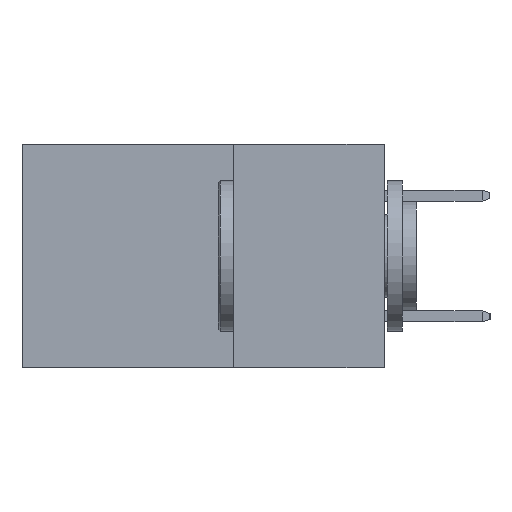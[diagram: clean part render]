
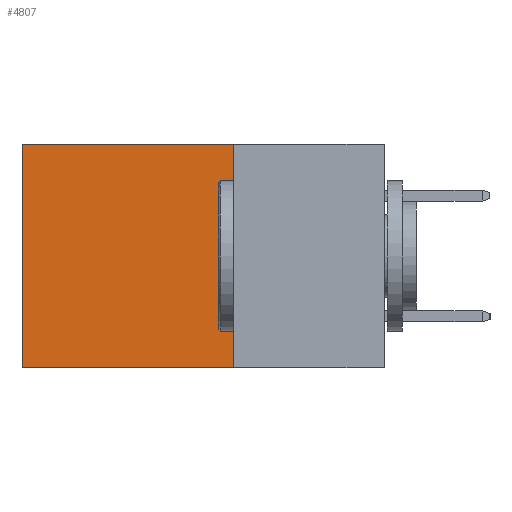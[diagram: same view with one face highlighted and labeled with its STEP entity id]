
A CAD part, left-side view. The second image highlights one B-rep face of the part: STEP entity #4807.
In plain terms, the highlighted planar face has unit normal (-1, 0, 0).
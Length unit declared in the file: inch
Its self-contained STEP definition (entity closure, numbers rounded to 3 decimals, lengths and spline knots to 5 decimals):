
#549 = EDGE_LOOP ( 'NONE', ( #6745, #1551, #2365, #1189 ) ) ;
#686 = DIRECTION ( 'NONE',  ( 0., 1., 0. ) ) ;
#787 = CARTESIAN_POINT ( 'NONE',  ( 0.2615, 0.25, 0. ) ) ;
#834 = FACE_OUTER_BOUND ( 'NONE', #549, .T. ) ;
#1189 = ORIENTED_EDGE ( 'NONE', *, *, #6927, .T. ) ;
#1272 = LINE ( 'NONE', #2302, #10806 ) ;
#1416 = CARTESIAN_POINT ( 'NONE',  ( 0.2615, 0.6, 0. ) ) ;
#1425 = AXIS2_PLACEMENT_3D ( 'NONE', #8714, #7562, #7513 ) ;
#1551 = ORIENTED_EDGE ( 'NONE', *, *, #2370, .F. ) ;
#2302 = CARTESIAN_POINT ( 'NONE',  ( 0.2615, 0.25, -0.37 ) ) ;
#2365 = ORIENTED_EDGE ( 'NONE', *, *, #4646, .F. ) ;
#2370 = EDGE_CURVE ( 'NONE', #10012, #10763, #10169, .T. ) ;
#2589 = DIRECTION ( 'NONE',  ( 0., 0., -1. ) ) ;
#2961 = DIRECTION ( 'NONE',  ( 0., 1., 0. ) ) ;
#4421 = CARTESIAN_POINT ( 'NONE',  ( 0.2615, 0.25, 0. ) ) ;
#4634 = VERTEX_POINT ( 'NONE', #4421 ) ;
#4646 = EDGE_CURVE ( 'NONE', #4634, #10012, #1272, .T. ) ;
#4711 = DIRECTION ( 'NONE',  ( 0., 0., -1. ) ) ;
#4807 = ADVANCED_FACE ( 'NONE', ( #834 ), #8085, .F. ) ;
#4948 = LINE ( 'NONE', #787, #7271 ) ;
#6517 = CARTESIAN_POINT ( 'NONE',  ( 0.2615, 0.6, -0.37 ) ) ;
#6690 = CARTESIAN_POINT ( 'NONE',  ( 0.2615, 0.6, -0.37 ) ) ;
#6745 = ORIENTED_EDGE ( 'NONE', *, *, #7302, .T. ) ;
#6927 = EDGE_CURVE ( 'NONE', #4634, #8091, #4948, .T. ) ;
#7234 = CARTESIAN_POINT ( 'NONE',  ( 0.2615, 0.25, -0.37 ) ) ;
#7271 = VECTOR ( 'NONE', #686, 39.37008 ) ;
#7302 = EDGE_CURVE ( 'NONE', #8091, #10763, #9912, .T. ) ;
#7513 = DIRECTION ( 'NONE',  ( 0., 0., -1. ) ) ;
#7562 = DIRECTION ( 'NONE',  ( 1., 0., 0. ) ) ;
#8054 = VECTOR ( 'NONE', #2961, 39.37008 ) ;
#8085 = PLANE ( 'NONE',  #1425 ) ;
#8091 = VERTEX_POINT ( 'NONE', #1416 ) ;
#8714 = CARTESIAN_POINT ( 'NONE',  ( 0.2615, 0.25, -0.37 ) ) ;
#9417 = VECTOR ( 'NONE', #4711, 39.37008 ) ;
#9766 = CARTESIAN_POINT ( 'NONE',  ( 0.2615, 0.25, -0.37 ) ) ;
#9912 = LINE ( 'NONE', #6690, #9417 ) ;
#10012 = VERTEX_POINT ( 'NONE', #7234 ) ;
#10169 = LINE ( 'NONE', #9766, #8054 ) ;
#10763 = VERTEX_POINT ( 'NONE', #6517 ) ;
#10806 = VECTOR ( 'NONE', #2589, 39.37008 ) ;
